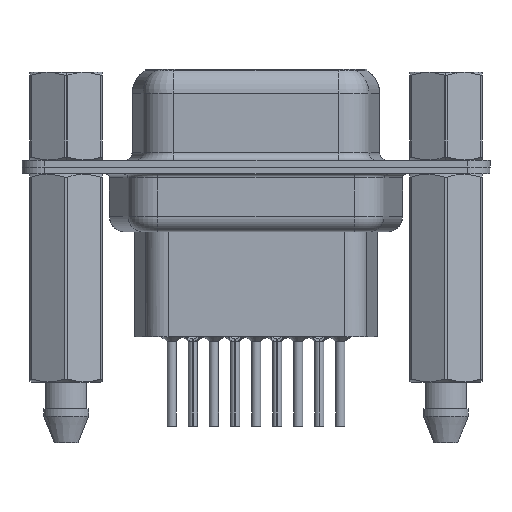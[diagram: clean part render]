
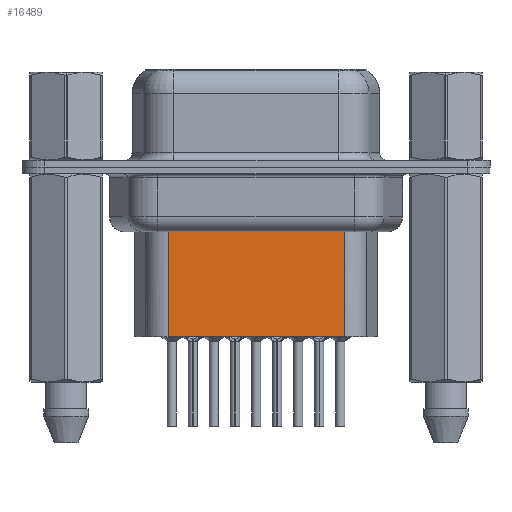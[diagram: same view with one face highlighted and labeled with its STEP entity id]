
A CAD part, front view. The second image highlights one B-rep face of the part: STEP entity #16489.
In plain terms, the highlighted planar face has unit normal (0, -1, 0).
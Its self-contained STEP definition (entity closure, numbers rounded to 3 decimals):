
#61 = ORIENTED_EDGE ( 'NONE', *, *, #19670, .T. ) ;
#251 = VECTOR ( 'NONE', #25271, 1000. ) ;
#587 = CARTESIAN_POINT ( 'NONE',  ( 6.706, -3.5, -3.1 ) ) ;
#597 = VECTOR ( 'NONE', #22290, 1000. ) ;
#679 = VERTEX_POINT ( 'NONE', #25782 ) ;
#858 = LINE ( 'NONE', #587, #597 ) ;
#1217 = CARTESIAN_POINT ( 'NONE',  ( 6.706, -3.5, -11.15 ) ) ;
#1917 = PLANE ( 'NONE',  #2994 ) ;
#2334 = DIRECTION ( 'NONE',  ( 1., 0., 0. ) ) ;
#2620 = VERTEX_POINT ( 'NONE', #8924 ) ;
#2994 = AXIS2_PLACEMENT_3D ( 'NONE', #27439, #14730, #2334 ) ;
#3819 = CARTESIAN_POINT ( 'NONE',  ( 18.294, -3.5, -3.1 ) ) ;
#5511 = CARTESIAN_POINT ( 'NONE',  ( 6.459, -3.5, -4.097 ) ) ;
#7852 = DIRECTION ( 'NONE',  ( -1., 0., 0. ) ) ;
#8514 = VECTOR ( 'NONE', #7852, 1000. ) ;
#8924 = CARTESIAN_POINT ( 'NONE',  ( 18.294, -3.5, -4.097 ) ) ;
#9804 = EDGE_CURVE ( 'NONE', #9876, #20584, #858, .T. ) ;
#9876 = VERTEX_POINT ( 'NONE', #16154 ) ;
#10208 = DIRECTION ( 'NONE',  ( 0., 0., -1. ) ) ;
#10608 = ORIENTED_EDGE ( 'NONE', *, *, #12015, .F. ) ;
#10659 = LINE ( 'NONE', #22899, #251 ) ;
#10981 = FACE_OUTER_BOUND ( 'NONE', #26152, .T. ) ;
#12015 = EDGE_CURVE ( 'NONE', #679, #20584, #10659, .T. ) ;
#14730 = DIRECTION ( 'NONE',  ( 0., -1., 0. ) ) ;
#16154 = CARTESIAN_POINT ( 'NONE',  ( 6.706, -3.5, -4.097 ) ) ;
#16450 = LINE ( 'NONE', #3819, #22764 ) ;
#16489 = ADVANCED_FACE ( 'NONE', ( #10981 ), #1917, .T. ) ;
#19670 = EDGE_CURVE ( 'NONE', #2620, #9876, #22327, .T. ) ;
#20584 = VERTEX_POINT ( 'NONE', #1217 ) ;
#20631 = ORIENTED_EDGE ( 'NONE', *, *, #9804, .T. ) ;
#22290 = DIRECTION ( 'NONE',  ( 0., 0., -1. ) ) ;
#22327 = LINE ( 'NONE', #5511, #8514 ) ;
#22764 = VECTOR ( 'NONE', #10208, 1000. ) ;
#22899 = CARTESIAN_POINT ( 'NONE',  ( 6.706, -3.5, -11.15 ) ) ;
#25271 = DIRECTION ( 'NONE',  ( -1., 0., 0. ) ) ;
#25782 = CARTESIAN_POINT ( 'NONE',  ( 18.294, -3.5, -11.15 ) ) ;
#25872 = EDGE_CURVE ( 'NONE', #2620, #679, #16450, .T. ) ;
#26152 = EDGE_LOOP ( 'NONE', ( #27041, #61, #20631, #10608 ) ) ;
#27041 = ORIENTED_EDGE ( 'NONE', *, *, #25872, .F. ) ;
#27439 = CARTESIAN_POINT ( 'NONE',  ( 6.706, -3.5, -3.1 ) ) ;
